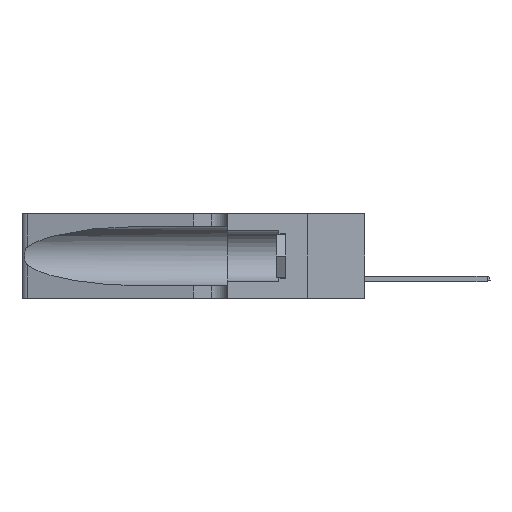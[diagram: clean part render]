
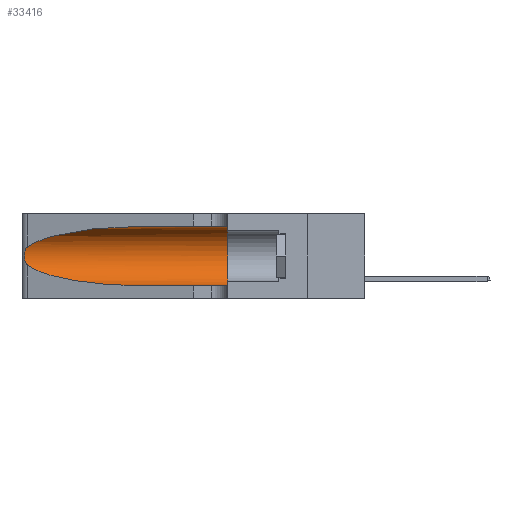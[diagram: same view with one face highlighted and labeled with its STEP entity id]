
A CAD part, left-side view. The second image highlights one B-rep face of the part: STEP entity #33416.
In plain terms, the highlighted cylindrical face has radius 3.308 mm (diameter 6.617 mm), a partial arc.
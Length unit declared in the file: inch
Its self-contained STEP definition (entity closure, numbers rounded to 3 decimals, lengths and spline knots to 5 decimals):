
#245 = FACE_OUTER_BOUND ( 'NONE', #27717, .T. ) ;
#305 = CARTESIAN_POINT ( 'NONE',  ( 0.1305, 1.61858, 0.05475 ) ) ;
#1504 = CARTESIAN_POINT ( 'NONE',  ( 0.25555, 1.22994, 0.2215 ) ) ;
#1940 = CARTESIAN_POINT ( 'NONE',  ( 0.1305, 0.35, 0.05475 ) ) ;
#2342 = VERTEX_POINT ( 'NONE', #1940 ) ;
#2594 = CARTESIAN_POINT ( 'NONE',  ( 0.18966, 0.96281, 0.31525 ) ) ;
#2675 = VERTEX_POINT ( 'NONE', #4982 ) ;
#3021 = VECTOR ( 'NONE', #16657, 39.37008 ) ;
#3082 = CARTESIAN_POINT ( 'NONE',  ( 0.1305, 0.72297, 0.31525 ) ) ;
#3266 = DIRECTION ( 'NONE',  ( 0., -1., 0. ) ) ;
#4110 = CARTESIAN_POINT ( 'NONE',  ( 0.25555, 1.22993, 0.14849 ) ) ;
#4221 = CARTESIAN_POINT ( 'NONE',  ( 0.26017, 1.23833, 0.17102 ) ) ;
#4944 = CARTESIAN_POINT ( 'NONE',  ( 0.25487, 1.22718, 0.22369 ) ) ;
#4982 = CARTESIAN_POINT ( 'NONE',  ( 0.25487, 1.22718, 0.22369 ) ) ;
#5596 = EDGE_CURVE ( 'NONE', #20031, #2342, #21217, .T. ) ;
#9353 = CARTESIAN_POINT ( 'NONE',  ( 0.2373, 1.15595, 0.08982 ) ) ;
#9907 = CARTESIAN_POINT ( 'NONE',  ( 0.25787, 1.23484, 0.2124 ) ) ;
#10043 = CARTESIAN_POINT ( 'NONE',  ( 0.18966, 0.96281, 0.05475 ) ) ;
#10519 = CARTESIAN_POINT ( 'NONE',  ( 0.2373, 1.15595, 0.28018 ) ) ;
#10760 = DIRECTION ( 'NONE',  ( 0., 0., 1. ) ) ;
#10879 = DIRECTION ( 'NONE',  ( 0., 1., 0. ) ) ;
#11899 = EDGE_CURVE ( 'NONE', #2675, #20481, #27739, .T. ) ;
#12874 = CARTESIAN_POINT ( 'NONE',  ( 0.1305, 0.72297, 0.05475 ) ) ;
#13597 = AXIS2_PLACEMENT_3D ( 'NONE', #30715, #17388, #20220 ) ;
#14904 = CARTESIAN_POINT ( 'NONE',  ( 0.25487, 1.22718, 0.14631 ) ) ;
#16532 = CARTESIAN_POINT ( 'NONE',  ( 0.1305, 1.61858, 0.31525 ) ) ;
#16657 = DIRECTION ( 'NONE',  ( 0., -1., 0. ) ) ;
#16861 = EDGE_CURVE ( 'NONE', #21310, #2675, #27287, .T. ) ;
#17388 = DIRECTION ( 'NONE',  ( 0., -1., 0. ) ) ;
#17708 = ORIENTED_EDGE ( 'NONE', *, *, #25824, .F. ) ;
#18948 = ORIENTED_EDGE ( 'NONE', *, *, #11899, .T. ) ;
#19039 = AXIS2_PLACEMENT_3D ( 'NONE', #32599, #10879, #10760 ) ;
#20031 = VERTEX_POINT ( 'NONE', #24093 ) ;
#20220 = DIRECTION ( 'NONE',  ( 0., 0., -1. ) ) ;
#20481 = VERTEX_POINT ( 'NONE', #34328 ) ;
#20563 = CARTESIAN_POINT ( 'NONE',  ( 0.26018, 1.23835, 0.19895 ) ) ;
#20762 = VECTOR ( 'NONE', #3266, 39.37008 ) ;
#21217 = LINE ( 'NONE', #305, #3021 ) ;
#21310 = VERTEX_POINT ( 'NONE', #3082 ) ;
#22845 = CARTESIAN_POINT ( 'NONE',  ( 0.25487, 1.22718, 0.14631 ) ) ;
#22941 = CARTESIAN_POINT ( 'NONE',  ( 0.25854, 1.2359, 0.20912 ) ) ;
#23174 = CARTESIAN_POINT ( 'NONE',  ( 0.25789, 1.23486, 0.15765 ) ) ;
#24093 = CARTESIAN_POINT ( 'NONE',  ( 0.1305, 0.72297, 0.05475 ) ) ;
#24828 = CIRCLE ( 'NONE', #19039, 0.13025 ) ;
#25653 = CARTESIAN_POINT ( 'NONE',  ( 0.26075, 1.23896, 0.178 ) ) ;
#25824 = EDGE_CURVE ( 'NONE', #21310, #26660, #33838, .T. ) ;
#26108 = CARTESIAN_POINT ( 'NONE',  ( 0.25639, 1.23184, 0.21858 ) ) ;
#26660 = VERTEX_POINT ( 'NONE', #27397 ) ;
#27287 =( BOUNDED_CURVE ( )  B_SPLINE_CURVE ( 3, ( #31907, #2594, #10519, #4944 ),
 .UNSPECIFIED., .F., .T. ) 
 B_SPLINE_CURVE_WITH_KNOTS ( ( 4, 4 ),
 ( 1.5708, 2.84003 ),
 .UNSPECIFIED. ) 
 CURVE ( )  GEOMETRIC_REPRESENTATION_ITEM ( )  RATIONAL_B_SPLINE_CURVE ( ( 1., 0.87, 0.87, 1. ) ) 
 REPRESENTATION_ITEM ( '' )  );
#27397 = CARTESIAN_POINT ( 'NONE',  ( 0.1305, 0.35, 0.31525 ) ) ;
#27717 = EDGE_LOOP ( 'NONE', ( #34124, #18948, #34381, #35027, #29706, #17708 ) ) ;
#27739 = B_SPLINE_CURVE_WITH_KNOTS ( 'NONE', 3,
 ( #31413, #1504, #26108, #9907, #22941, #20563, #33991, #25653, #4221, #31067, #23174, #28587, #4110, #14904 ),
 .UNSPECIFIED., .F., .F.,
 ( 4, 2, 2, 2, 2, 2, 4 ),
 ( 0., 0.00027, 0.00053, 0.00107, 0.0016, 0.00187, 0.00214 ),
 .UNSPECIFIED. ) ;
#28587 = CARTESIAN_POINT ( 'NONE',  ( 0.25639, 1.23186, 0.15144 ) ) ;
#29706 = ORIENTED_EDGE ( 'NONE', *, *, #33034, .F. ) ;
#30715 = CARTESIAN_POINT ( 'NONE',  ( 0.1305, 1.61858, 0.185 ) ) ;
#30963 =( BOUNDED_CURVE ( )  B_SPLINE_CURVE ( 3, ( #22845, #9353, #10043, #12874 ),
 .UNSPECIFIED., .F., .T. ) 
 B_SPLINE_CURVE_WITH_KNOTS ( ( 4, 4 ),
 ( 3.44316, 4.71239 ),
 .UNSPECIFIED. ) 
 CURVE ( )  GEOMETRIC_REPRESENTATION_ITEM ( )  RATIONAL_B_SPLINE_CURVE ( ( 1., 0.87, 0.87, 1. ) ) 
 REPRESENTATION_ITEM ( '' )  );
#31067 = CARTESIAN_POINT ( 'NONE',  ( 0.25856, 1.23593, 0.16098 ) ) ;
#31413 = CARTESIAN_POINT ( 'NONE',  ( 0.25487, 1.22718, 0.22369 ) ) ;
#31521 = EDGE_CURVE ( 'NONE', #20481, #20031, #30963, .T. ) ;
#31907 = CARTESIAN_POINT ( 'NONE',  ( 0.1305, 0.72297, 0.31525 ) ) ;
#32599 = CARTESIAN_POINT ( 'NONE',  ( 0.1305, 0.35, 0.185 ) ) ;
#33034 = EDGE_CURVE ( 'NONE', #26660, #2342, #24828, .T. ) ;
#33251 = CYLINDRICAL_SURFACE ( 'NONE', #13597, 0.13025 ) ;
#33416 = ADVANCED_FACE ( 'NONE', ( #245 ), #33251, .F. ) ;
#33838 = LINE ( 'NONE', #16532, #20762 ) ;
#33991 = CARTESIAN_POINT ( 'NONE',  ( 0.26075, 1.23896, 0.19203 ) ) ;
#34124 = ORIENTED_EDGE ( 'NONE', *, *, #16861, .T. ) ;
#34328 = CARTESIAN_POINT ( 'NONE',  ( 0.25487, 1.22718, 0.14631 ) ) ;
#34381 = ORIENTED_EDGE ( 'NONE', *, *, #31521, .T. ) ;
#35027 = ORIENTED_EDGE ( 'NONE', *, *, #5596, .T. ) ;
